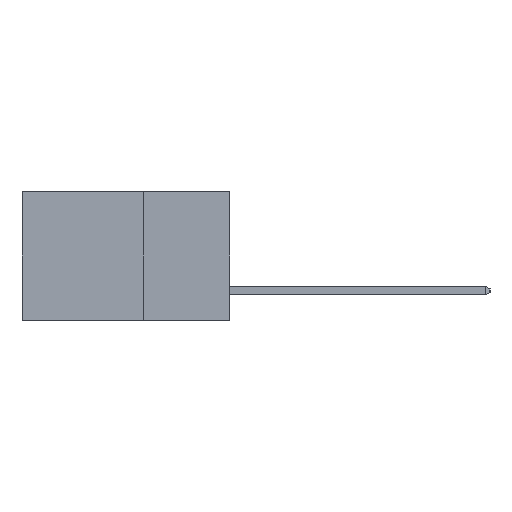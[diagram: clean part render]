
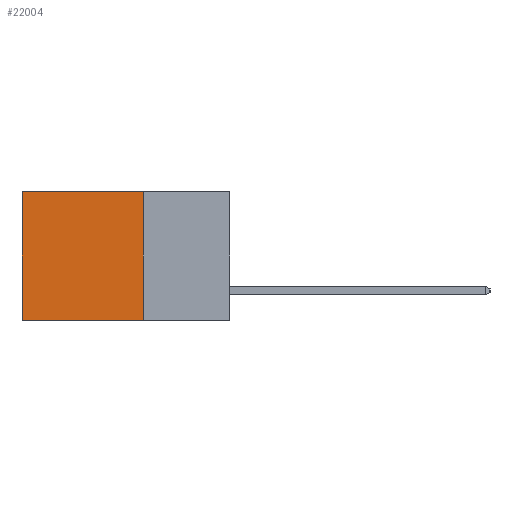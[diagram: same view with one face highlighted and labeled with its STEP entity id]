
A CAD part, left-side view. The second image highlights one B-rep face of the part: STEP entity #22004.
In plain terms, the highlighted planar face has unit normal (-1, 0, 0).
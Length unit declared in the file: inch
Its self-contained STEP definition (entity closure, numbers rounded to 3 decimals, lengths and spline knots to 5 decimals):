
#1121 = VECTOR ( 'NONE', #26168, 39.37008 ) ;
#1731 = LINE ( 'NONE', #10558, #18671 ) ;
#1806 = LINE ( 'NONE', #24047, #1121 ) ;
#1867 = DIRECTION ( 'NONE',  ( 0., 1., 0. ) ) ;
#2794 = ORIENTED_EDGE ( 'NONE', *, *, #23418, .F. ) ;
#3254 = CARTESIAN_POINT ( 'NONE',  ( 0.298, 0.25, -0.37 ) ) ;
#3762 = DIRECTION ( 'NONE',  ( 0., 0., -1. ) ) ;
#4690 = VECTOR ( 'NONE', #3762, 39.37008 ) ;
#5631 = PLANE ( 'NONE',  #11277 ) ;
#7770 = DIRECTION ( 'NONE',  ( 1., 0., 0. ) ) ;
#8034 = VERTEX_POINT ( 'NONE', #3254 ) ;
#8160 = LINE ( 'NONE', #27276, #13753 ) ;
#8284 = EDGE_CURVE ( 'NONE', #25373, #10668, #1731, .T. ) ;
#8802 = EDGE_CURVE ( 'NONE', #10885, #8034, #21670, .T. ) ;
#9741 = CARTESIAN_POINT ( 'NONE',  ( 0.298, 0.25, 0. ) ) ;
#10558 = CARTESIAN_POINT ( 'NONE',  ( 0.298, 0.6, 0. ) ) ;
#10668 = VERTEX_POINT ( 'NONE', #15338 ) ;
#10885 = VERTEX_POINT ( 'NONE', #9741 ) ;
#11277 = AXIS2_PLACEMENT_3D ( 'NONE', #11881, #7770, #22652 ) ;
#11881 = CARTESIAN_POINT ( 'NONE',  ( 0.298, 0.25, 0. ) ) ;
#13753 = VECTOR ( 'NONE', #1867, 39.37008 ) ;
#14315 = CARTESIAN_POINT ( 'NONE',  ( 0.298, 0.25, 0. ) ) ;
#14467 = EDGE_CURVE ( 'NONE', #10885, #25373, #1806, .T. ) ;
#15338 = CARTESIAN_POINT ( 'NONE',  ( 0.298, 0.6, -0.37 ) ) ;
#17981 = ORIENTED_EDGE ( 'NONE', *, *, #8802, .F. ) ;
#18536 = FACE_OUTER_BOUND ( 'NONE', #20749, .T. ) ;
#18671 = VECTOR ( 'NONE', #25444, 39.37008 ) ;
#19132 = ORIENTED_EDGE ( 'NONE', *, *, #14467, .T. ) ;
#20749 = EDGE_LOOP ( 'NONE', ( #23794, #2794, #17981, #19132 ) ) ;
#21670 = LINE ( 'NONE', #14315, #4690 ) ;
#22004 = ADVANCED_FACE ( 'NONE', ( #18536 ), #5631, .F. ) ;
#22652 = DIRECTION ( 'NONE',  ( 0., 0., -1. ) ) ;
#23418 = EDGE_CURVE ( 'NONE', #8034, #10668, #8160, .T. ) ;
#23794 = ORIENTED_EDGE ( 'NONE', *, *, #8284, .T. ) ;
#24047 = CARTESIAN_POINT ( 'NONE',  ( 0.298, 0.25, 0. ) ) ;
#24109 = CARTESIAN_POINT ( 'NONE',  ( 0.298, 0.6, 0. ) ) ;
#25373 = VERTEX_POINT ( 'NONE', #24109 ) ;
#25444 = DIRECTION ( 'NONE',  ( 0., 0., -1. ) ) ;
#26168 = DIRECTION ( 'NONE',  ( 0., 1., 0. ) ) ;
#27276 = CARTESIAN_POINT ( 'NONE',  ( 0.298, 0.25, -0.37 ) ) ;
